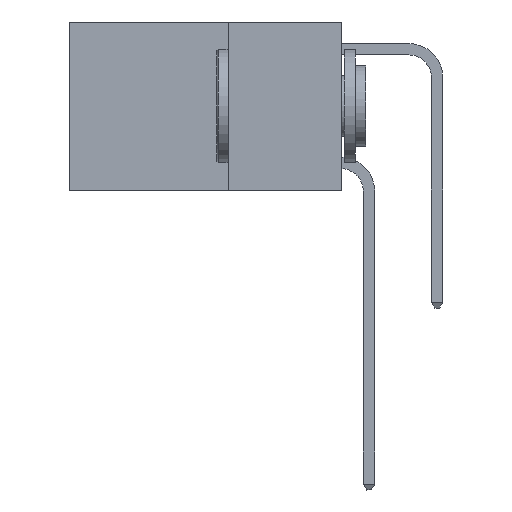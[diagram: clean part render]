
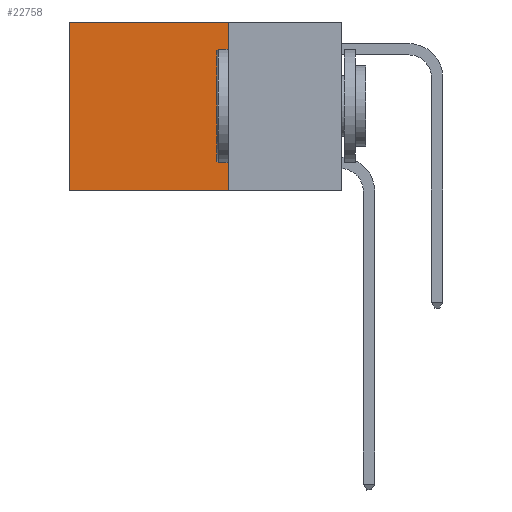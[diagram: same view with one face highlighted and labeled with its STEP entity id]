
A CAD part, left-side view. The second image highlights one B-rep face of the part: STEP entity #22758.
In plain terms, the highlighted planar face has unit normal (-1, 0, 0).
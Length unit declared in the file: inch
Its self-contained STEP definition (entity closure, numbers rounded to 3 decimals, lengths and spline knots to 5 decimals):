
#622 = EDGE_CURVE ( 'NONE', #8933, #12405, #18195, .T. ) ;
#627 = CARTESIAN_POINT ( 'NONE',  ( 0.2625, 0.25, 0. ) ) ;
#1480 = VECTOR ( 'NONE', #28337, 39.37008 ) ;
#2066 = EDGE_CURVE ( 'NONE', #33814, #23092, #12161, .T. ) ;
#2109 = ORIENTED_EDGE ( 'NONE', *, *, #21603, .F. ) ;
#2701 = VECTOR ( 'NONE', #10509, 39.37008 ) ;
#4657 = ORIENTED_EDGE ( 'NONE', *, *, #17492, .T. ) ;
#6089 = CARTESIAN_POINT ( 'NONE',  ( 0.2625, 0.25, -0.37 ) ) ;
#7019 = LINE ( 'NONE', #17666, #1480 ) ;
#8037 = CARTESIAN_POINT ( 'NONE',  ( 0.2625, 0.6, 0. ) ) ;
#8933 = VERTEX_POINT ( 'NONE', #18258 ) ;
#9126 = VECTOR ( 'NONE', #20473, 39.37008 ) ;
#9534 = DIRECTION ( 'NONE',  ( 0., 0., -1. ) ) ;
#10509 = DIRECTION ( 'NONE',  ( 0., 0., -1. ) ) ;
#12161 = LINE ( 'NONE', #22792, #30216 ) ;
#12405 = VERTEX_POINT ( 'NONE', #6089 ) ;
#14734 = LINE ( 'NONE', #33757, #9126 ) ;
#16315 = PLANE ( 'NONE',  #28836 ) ;
#16827 = FACE_OUTER_BOUND ( 'NONE', #25639, .T. ) ;
#17492 = EDGE_CURVE ( 'NONE', #8933, #33814, #14734, .T. ) ;
#17666 = CARTESIAN_POINT ( 'NONE',  ( 0.2625, 0.25, -0.37 ) ) ;
#17865 = CARTESIAN_POINT ( 'NONE',  ( 0.2625, 0.25, 0. ) ) ;
#18195 = LINE ( 'NONE', #17865, #2701 ) ;
#18258 = CARTESIAN_POINT ( 'NONE',  ( 0.2625, 0.25, 0. ) ) ;
#20473 = DIRECTION ( 'NONE',  ( 0., 1., 0. ) ) ;
#21603 = EDGE_CURVE ( 'NONE', #12405, #23092, #7019, .T. ) ;
#22758 = ADVANCED_FACE ( 'NONE', ( #16827 ), #16315, .F. ) ;
#22792 = CARTESIAN_POINT ( 'NONE',  ( 0.2625, 0.6, 0. ) ) ;
#23092 = VERTEX_POINT ( 'NONE', #27441 ) ;
#25639 = EDGE_LOOP ( 'NONE', ( #29389, #2109, #31320, #4657 ) ) ;
#27441 = CARTESIAN_POINT ( 'NONE',  ( 0.2625, 0.6, -0.37 ) ) ;
#28337 = DIRECTION ( 'NONE',  ( 0., 1., 0. ) ) ;
#28836 = AXIS2_PLACEMENT_3D ( 'NONE', #627, #32349, #29576 ) ;
#29389 = ORIENTED_EDGE ( 'NONE', *, *, #2066, .T. ) ;
#29576 = DIRECTION ( 'NONE',  ( 0., 0., -1. ) ) ;
#30216 = VECTOR ( 'NONE', #9534, 39.37008 ) ;
#31320 = ORIENTED_EDGE ( 'NONE', *, *, #622, .F. ) ;
#32349 = DIRECTION ( 'NONE',  ( 1., 0., 0. ) ) ;
#33757 = CARTESIAN_POINT ( 'NONE',  ( 0.2625, 0.25, 0. ) ) ;
#33814 = VERTEX_POINT ( 'NONE', #8037 ) ;
